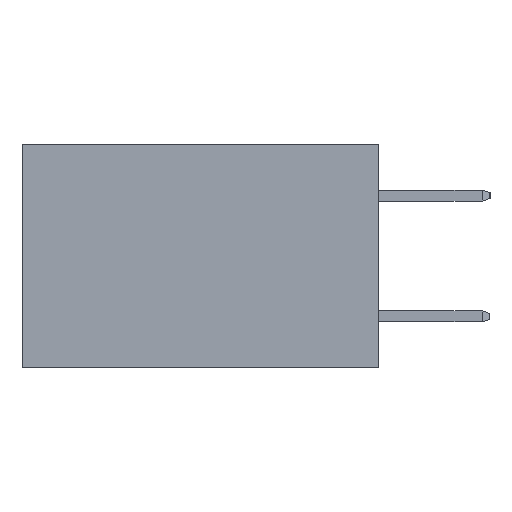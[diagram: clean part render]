
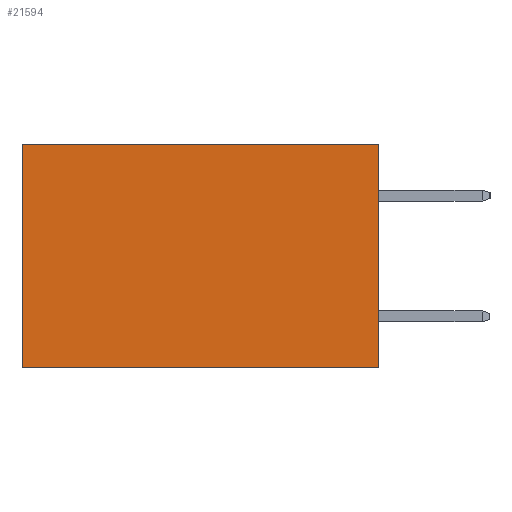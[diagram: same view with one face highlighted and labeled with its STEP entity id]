
A CAD part, left-side view. The second image highlights one B-rep face of the part: STEP entity #21594.
In plain terms, the highlighted planar face has unit normal (-1, 0, 0).
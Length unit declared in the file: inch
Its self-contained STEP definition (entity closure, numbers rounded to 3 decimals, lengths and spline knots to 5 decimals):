
#1611 = DIRECTION ( 'NONE',  ( 0., 1., 0. ) ) ;
#2889 = ORIENTED_EDGE ( 'NONE', *, *, #12763, .F. ) ;
#3366 = VECTOR ( 'NONE', #22692, 39.37008 ) ;
#4147 = VECTOR ( 'NONE', #1611, 39.37008 ) ;
#4155 = EDGE_CURVE ( 'NONE', #28891, #13311, #29549, .T. ) ;
#4346 = EDGE_CURVE ( 'NONE', #12552, #7676, #23470, .T. ) ;
#5703 = EDGE_LOOP ( 'NONE', ( #16496, #2889, #17682, #30582 ) ) ;
#7676 = VERTEX_POINT ( 'NONE', #23322 ) ;
#8387 = VECTOR ( 'NONE', #28012, 39.37008 ) ;
#11672 = DIRECTION ( 'NONE',  ( 1., 0., 0. ) ) ;
#11922 = DIRECTION ( 'NONE',  ( 0., 0., -1. ) ) ;
#12464 = CARTESIAN_POINT ( 'NONE',  ( 0.277, 0.59, 0. ) ) ;
#12552 = VERTEX_POINT ( 'NONE', #12464 ) ;
#12763 = EDGE_CURVE ( 'NONE', #13311, #7676, #27963, .T. ) ;
#13311 = VERTEX_POINT ( 'NONE', #27453 ) ;
#14037 = CARTESIAN_POINT ( 'NONE',  ( 0.277, 0.59, -0.37 ) ) ;
#16496 = ORIENTED_EDGE ( 'NONE', *, *, #4346, .T. ) ;
#16975 = VECTOR ( 'NONE', #11922, 39.37008 ) ;
#17365 = LINE ( 'NONE', #28681, #4147 ) ;
#17682 = ORIENTED_EDGE ( 'NONE', *, *, #4155, .F. ) ;
#21294 = PLANE ( 'NONE',  #25455 ) ;
#21594 = ADVANCED_FACE ( 'NONE', ( #23283 ), #21294, .F. ) ;
#22692 = DIRECTION ( 'NONE',  ( 0., 0., -1. ) ) ;
#22963 = CARTESIAN_POINT ( 'NONE',  ( 0.277, 0., 0. ) ) ;
#23283 = FACE_OUTER_BOUND ( 'NONE', #5703, .T. ) ;
#23322 = CARTESIAN_POINT ( 'NONE',  ( 0.277, 0.59, -0.37 ) ) ;
#23470 = LINE ( 'NONE', #14037, #16975 ) ;
#23731 = CARTESIAN_POINT ( 'NONE',  ( 0.277, 0., -0.37 ) ) ;
#23837 = CARTESIAN_POINT ( 'NONE',  ( 0.277, 0., -0.37 ) ) ;
#25328 = EDGE_CURVE ( 'NONE', #28891, #12552, #17365, .T. ) ;
#25455 = AXIS2_PLACEMENT_3D ( 'NONE', #23837, #11672, #28704 ) ;
#25567 = CARTESIAN_POINT ( 'NONE',  ( 0.277, 0., -0.37 ) ) ;
#27453 = CARTESIAN_POINT ( 'NONE',  ( 0.277, 0., -0.37 ) ) ;
#27963 = LINE ( 'NONE', #25567, #8387 ) ;
#28012 = DIRECTION ( 'NONE',  ( 0., 1., 0. ) ) ;
#28681 = CARTESIAN_POINT ( 'NONE',  ( 0.277, 0., 0. ) ) ;
#28704 = DIRECTION ( 'NONE',  ( 0., 0., -1. ) ) ;
#28891 = VERTEX_POINT ( 'NONE', #22963 ) ;
#29549 = LINE ( 'NONE', #23731, #3366 ) ;
#30582 = ORIENTED_EDGE ( 'NONE', *, *, #25328, .T. ) ;
